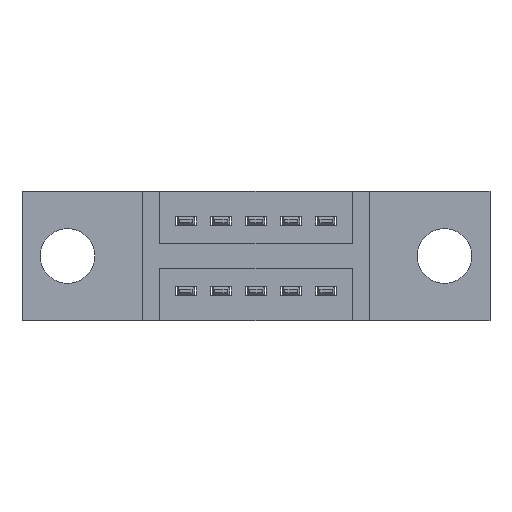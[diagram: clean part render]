
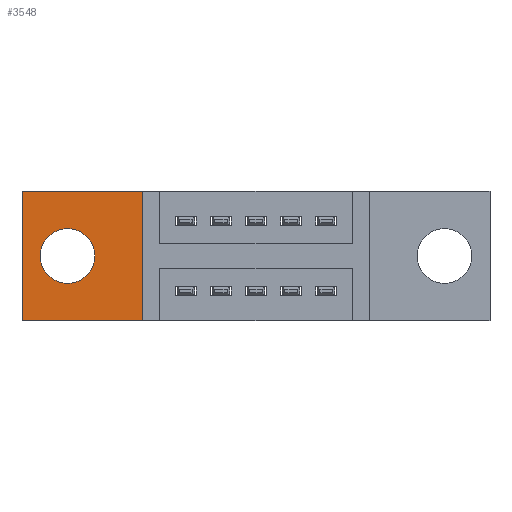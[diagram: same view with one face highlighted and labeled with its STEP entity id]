
A CAD part, front view. The second image highlights one B-rep face of the part: STEP entity #3548.
In plain terms, the highlighted planar face has unit normal (0, -1, 0).
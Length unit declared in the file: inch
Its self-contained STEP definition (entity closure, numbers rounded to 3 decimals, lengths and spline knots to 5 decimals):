
#29 = DIRECTION ( 'NONE',  ( 0., -1., 0. ) ) ;
#153 = EDGE_CURVE ( 'NONE', #6077, #5815, #3345, .T. ) ;
#271 = EDGE_LOOP ( 'NONE', ( #4207, #3574 ) ) ;
#312 = CIRCLE ( 'NONE', #7975, 0.078 ) ;
#407 = VERTEX_POINT ( 'NONE', #1684 ) ;
#452 = VECTOR ( 'NONE', #8043, 39.37008 ) ;
#557 = FACE_OUTER_BOUND ( 'NONE', #1818, .T. ) ;
#599 = CARTESIAN_POINT ( 'NONE',  ( 0., 0.17, 0. ) ) ;
#891 = LINE ( 'NONE', #2324, #452 ) ;
#1117 = EDGE_CURVE ( 'NONE', #407, #6077, #2197, .T. ) ;
#1684 = CARTESIAN_POINT ( 'NONE',  ( 0.3425, 0.17, -0.37 ) ) ;
#1818 = EDGE_LOOP ( 'NONE', ( #8417, #3586, #5148, #3739 ) ) ;
#1836 = DIRECTION ( 'NONE',  ( -1., 0., 0. ) ) ;
#1881 = LINE ( 'NONE', #5489, #4391 ) ;
#2047 = CARTESIAN_POINT ( 'NONE',  ( 0.13, 0.17, -0.107 ) ) ;
#2197 = LINE ( 'NONE', #4195, #5219 ) ;
#2324 = CARTESIAN_POINT ( 'NONE',  ( 0., 0.17, -0.37 ) ) ;
#2458 = EDGE_CURVE ( 'NONE', #7256, #8755, #8847, .T. ) ;
#2855 = CARTESIAN_POINT ( 'NONE',  ( 0., 0.17, 0. ) ) ;
#3019 = EDGE_CURVE ( 'NONE', #4683, #407, #891, .T. ) ;
#3345 = LINE ( 'NONE', #599, #6391 ) ;
#3548 = ADVANCED_FACE ( 'NONE', ( #6998, #557 ), #5578, .T. ) ;
#3574 = ORIENTED_EDGE ( 'NONE', *, *, #2458, .F. ) ;
#3586 = ORIENTED_EDGE ( 'NONE', *, *, #3019, .T. ) ;
#3739 = ORIENTED_EDGE ( 'NONE', *, *, #153, .T. ) ;
#3772 = AXIS2_PLACEMENT_3D ( 'NONE', #3955, #6821, #4327 ) ;
#3955 = CARTESIAN_POINT ( 'NONE',  ( 0., 0.17, -0.37 ) ) ;
#4195 = CARTESIAN_POINT ( 'NONE',  ( 0.3425, 0.17, 0. ) ) ;
#4207 = ORIENTED_EDGE ( 'NONE', *, *, #5487, .F. ) ;
#4327 = DIRECTION ( 'NONE',  ( 0., 0., -1. ) ) ;
#4391 = VECTOR ( 'NONE', #7741, 39.37008 ) ;
#4683 = VERTEX_POINT ( 'NONE', #6116 ) ;
#5148 = ORIENTED_EDGE ( 'NONE', *, *, #1117, .T. ) ;
#5219 = VECTOR ( 'NONE', #5600, 39.37008 ) ;
#5270 = EDGE_CURVE ( 'NONE', #5815, #4683, #1881, .T. ) ;
#5463 = CARTESIAN_POINT ( 'NONE',  ( 0.3425, 0.17, 0. ) ) ;
#5487 = EDGE_CURVE ( 'NONE', #8755, #7256, #312, .T. ) ;
#5489 = CARTESIAN_POINT ( 'NONE',  ( 0., 0.17, 0. ) ) ;
#5578 = PLANE ( 'NONE',  #3772 ) ;
#5600 = DIRECTION ( 'NONE',  ( 0., 0., 1. ) ) ;
#5815 = VERTEX_POINT ( 'NONE', #2855 ) ;
#5863 = DIRECTION ( 'NONE',  ( 0., 0., -1. ) ) ;
#5915 = CARTESIAN_POINT ( 'NONE',  ( 0.13, 0.17, -0.185 ) ) ;
#6042 = CARTESIAN_POINT ( 'NONE',  ( 0.13, 0.17, -0.263 ) ) ;
#6077 = VERTEX_POINT ( 'NONE', #5463 ) ;
#6116 = CARTESIAN_POINT ( 'NONE',  ( 0., 0.17, -0.37 ) ) ;
#6391 = VECTOR ( 'NONE', #1836, 39.37008 ) ;
#6514 = DIRECTION ( 'NONE',  ( 0., 0., -1. ) ) ;
#6821 = DIRECTION ( 'NONE',  ( 0., -1., 0. ) ) ;
#6998 = FACE_BOUND ( 'NONE', #271, .T. ) ;
#7256 = VERTEX_POINT ( 'NONE', #6042 ) ;
#7741 = DIRECTION ( 'NONE',  ( 0., 0., -1. ) ) ;
#7958 = CARTESIAN_POINT ( 'NONE',  ( 0.13, 0.17, -0.185 ) ) ;
#7975 = AXIS2_PLACEMENT_3D ( 'NONE', #5915, #8861, #5863 ) ;
#8043 = DIRECTION ( 'NONE',  ( 1., 0., 0. ) ) ;
#8417 = ORIENTED_EDGE ( 'NONE', *, *, #5270, .T. ) ;
#8755 = VERTEX_POINT ( 'NONE', #2047 ) ;
#8847 = CIRCLE ( 'NONE', #9149, 0.078 ) ;
#8861 = DIRECTION ( 'NONE',  ( 0., -1., 0. ) ) ;
#9149 = AXIS2_PLACEMENT_3D ( 'NONE', #7958, #29, #6514 ) ;
